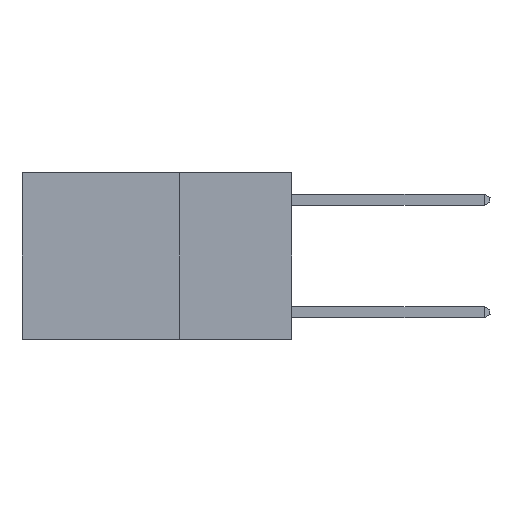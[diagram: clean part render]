
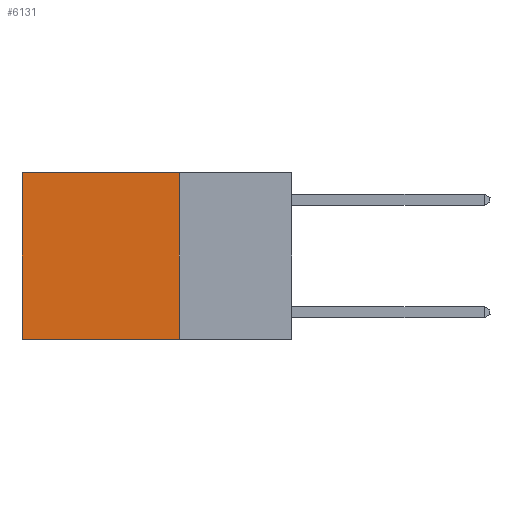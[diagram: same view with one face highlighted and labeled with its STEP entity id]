
A CAD part, left-side view. The second image highlights one B-rep face of the part: STEP entity #6131.
In plain terms, the highlighted planar face has unit normal (-1, 0, 0).
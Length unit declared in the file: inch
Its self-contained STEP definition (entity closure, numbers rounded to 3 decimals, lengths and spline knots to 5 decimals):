
#512 = ORIENTED_EDGE ( 'NONE', *, *, #4541, .T. ) ;
#776 = EDGE_CURVE ( 'NONE', #5133, #7940, #15704, .T. ) ;
#922 = DIRECTION ( 'NONE',  ( 1., 0., 0. ) ) ;
#1362 = CARTESIAN_POINT ( 'NONE',  ( 0.2625, 0.25, -0.37 ) ) ;
#1389 = DIRECTION ( 'NONE',  ( 0., 0., -1. ) ) ;
#2607 = VECTOR ( 'NONE', #4904, 39.37008 ) ;
#2729 = LINE ( 'NONE', #8564, #11655 ) ;
#3870 = CARTESIAN_POINT ( 'NONE',  ( 0.2625, 0.25, -0.37 ) ) ;
#4541 = EDGE_CURVE ( 'NONE', #10489, #5133, #13612, .T. ) ;
#4556 = EDGE_CURVE ( 'NONE', #10489, #9720, #2729, .T. ) ;
#4904 = DIRECTION ( 'NONE',  ( 0., 1., 0. ) ) ;
#5133 = VERTEX_POINT ( 'NONE', #7838 ) ;
#5916 = CARTESIAN_POINT ( 'NONE',  ( 0.2625, 0.6, 0. ) ) ;
#5928 = PLANE ( 'NONE',  #14740 ) ;
#6131 = ADVANCED_FACE ( 'NONE', ( #7130 ), #5928, .F. ) ;
#6499 = CARTESIAN_POINT ( 'NONE',  ( 0.2625, 0.6, -0.37 ) ) ;
#7130 = FACE_OUTER_BOUND ( 'NONE', #10750, .T. ) ;
#7193 = CARTESIAN_POINT ( 'NONE',  ( 0.2625, 0.25, 0. ) ) ;
#7498 = DIRECTION ( 'NONE',  ( 0., 1., 0. ) ) ;
#7838 = CARTESIAN_POINT ( 'NONE',  ( 0.2625, 0.6, 0. ) ) ;
#7940 = VERTEX_POINT ( 'NONE', #6499 ) ;
#8564 = CARTESIAN_POINT ( 'NONE',  ( 0.2625, 0.25, 0. ) ) ;
#9720 = VERTEX_POINT ( 'NONE', #3870 ) ;
#10013 = CARTESIAN_POINT ( 'NONE',  ( 0.2625, 0.25, 0. ) ) ;
#10489 = VERTEX_POINT ( 'NONE', #7193 ) ;
#10750 = EDGE_LOOP ( 'NONE', ( #12296, #15768, #10886, #512 ) ) ;
#10886 = ORIENTED_EDGE ( 'NONE', *, *, #4556, .F. ) ;
#10904 = CARTESIAN_POINT ( 'NONE',  ( 0.2625, 0.25, 0. ) ) ;
#11655 = VECTOR ( 'NONE', #14904, 39.37008 ) ;
#12296 = ORIENTED_EDGE ( 'NONE', *, *, #776, .T. ) ;
#13478 = LINE ( 'NONE', #1362, #15267 ) ;
#13612 = LINE ( 'NONE', #10013, #2607 ) ;
#14740 = AXIS2_PLACEMENT_3D ( 'NONE', #10904, #922, #15806 ) ;
#14898 = EDGE_CURVE ( 'NONE', #9720, #7940, #13478, .T. ) ;
#14904 = DIRECTION ( 'NONE',  ( 0., 0., -1. ) ) ;
#15127 = VECTOR ( 'NONE', #1389, 39.37008 ) ;
#15267 = VECTOR ( 'NONE', #7498, 39.37008 ) ;
#15704 = LINE ( 'NONE', #5916, #15127 ) ;
#15768 = ORIENTED_EDGE ( 'NONE', *, *, #14898, .F. ) ;
#15806 = DIRECTION ( 'NONE',  ( 0., 0., -1. ) ) ;
